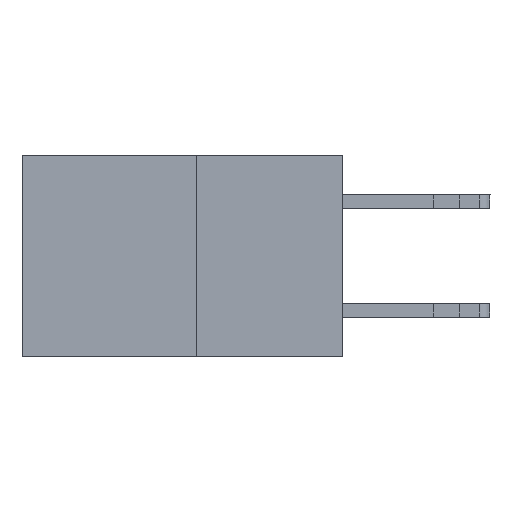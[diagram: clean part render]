
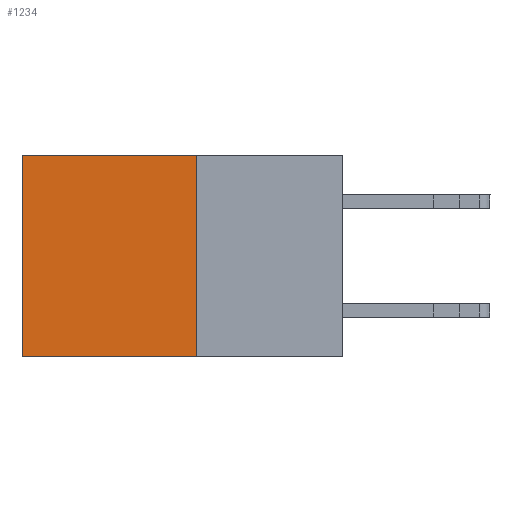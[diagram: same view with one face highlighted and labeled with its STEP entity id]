
A CAD part, left-side view. The second image highlights one B-rep face of the part: STEP entity #1234.
In plain terms, the highlighted planar face has unit normal (-1, 0, 0).
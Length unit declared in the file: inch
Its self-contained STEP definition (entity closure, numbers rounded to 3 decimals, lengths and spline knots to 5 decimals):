
#1234 = ADVANCED_FACE ( 'NONE', ( #4244 ), #10620, .F. ) ;
#1959 = EDGE_LOOP ( 'NONE', ( #17437, #19832, #19437, #13379 ) ) ;
#1963 = LINE ( 'NONE', #12979, #2363 ) ;
#2190 = EDGE_CURVE ( 'NONE', #8416, #16636, #13431, .T. ) ;
#2209 = DIRECTION ( 'NONE',  ( 0., 0., -1. ) ) ;
#2363 = VECTOR ( 'NONE', #15351, 39.37008 ) ;
#2692 = VECTOR ( 'NONE', #2209, 39.37008 ) ;
#2975 = VERTEX_POINT ( 'NONE', #18887 ) ;
#3623 = CARTESIAN_POINT ( 'NONE',  ( 0.277, 0.27, 0. ) ) ;
#3632 = EDGE_CURVE ( 'NONE', #2975, #15334, #12704, .T. ) ;
#4244 = FACE_OUTER_BOUND ( 'NONE', #1959, .T. ) ;
#6860 = CARTESIAN_POINT ( 'NONE',  ( 0.277, 0.27, -0.37 ) ) ;
#7551 = VECTOR ( 'NONE', #18065, 39.37008 ) ;
#8416 = VERTEX_POINT ( 'NONE', #3623 ) ;
#9254 = CARTESIAN_POINT ( 'NONE',  ( 0.277, 0.27, -0.37 ) ) ;
#10504 = DIRECTION ( 'NONE',  ( 0., 0., -1. ) ) ;
#10620 = PLANE ( 'NONE',  #17946 ) ;
#10731 = VECTOR ( 'NONE', #16621, 39.37008 ) ;
#11562 = CARTESIAN_POINT ( 'NONE',  ( 0.277, 0.59, -0.37 ) ) ;
#11772 = CARTESIAN_POINT ( 'NONE',  ( 0.277, 0.59, -0.37 ) ) ;
#12704 = LINE ( 'NONE', #11562, #2692 ) ;
#12979 = CARTESIAN_POINT ( 'NONE',  ( 0.277, 0.27, 0. ) ) ;
#13379 = ORIENTED_EDGE ( 'NONE', *, *, #15923, .T. ) ;
#13431 = LINE ( 'NONE', #19707, #10731 ) ;
#13686 = DIRECTION ( 'NONE',  ( 1., 0., 0. ) ) ;
#14947 = EDGE_CURVE ( 'NONE', #16636, #15334, #19516, .T. ) ;
#15334 = VERTEX_POINT ( 'NONE', #11772 ) ;
#15351 = DIRECTION ( 'NONE',  ( 0., 1., 0. ) ) ;
#15923 = EDGE_CURVE ( 'NONE', #8416, #2975, #1963, .T. ) ;
#16617 = CARTESIAN_POINT ( 'NONE',  ( 0.277, 0.27, -0.37 ) ) ;
#16621 = DIRECTION ( 'NONE',  ( 0., 0., -1. ) ) ;
#16636 = VERTEX_POINT ( 'NONE', #16617 ) ;
#17437 = ORIENTED_EDGE ( 'NONE', *, *, #3632, .T. ) ;
#17946 = AXIS2_PLACEMENT_3D ( 'NONE', #9254, #13686, #10504 ) ;
#18065 = DIRECTION ( 'NONE',  ( 0., 1., 0. ) ) ;
#18887 = CARTESIAN_POINT ( 'NONE',  ( 0.277, 0.59, 0. ) ) ;
#19437 = ORIENTED_EDGE ( 'NONE', *, *, #2190, .F. ) ;
#19516 = LINE ( 'NONE', #6860, #7551 ) ;
#19707 = CARTESIAN_POINT ( 'NONE',  ( 0.277, 0.27, -0.37 ) ) ;
#19832 = ORIENTED_EDGE ( 'NONE', *, *, #14947, .F. ) ;
